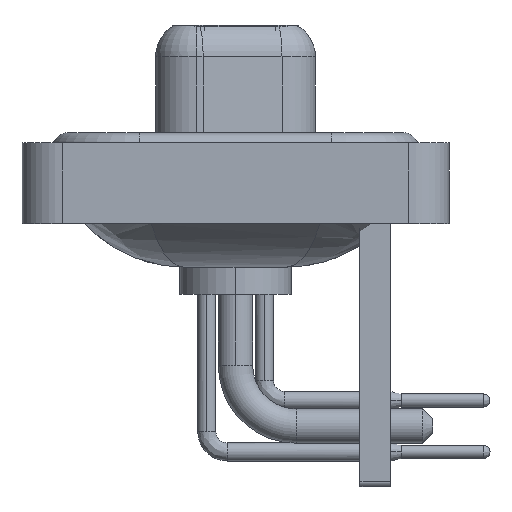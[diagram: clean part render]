
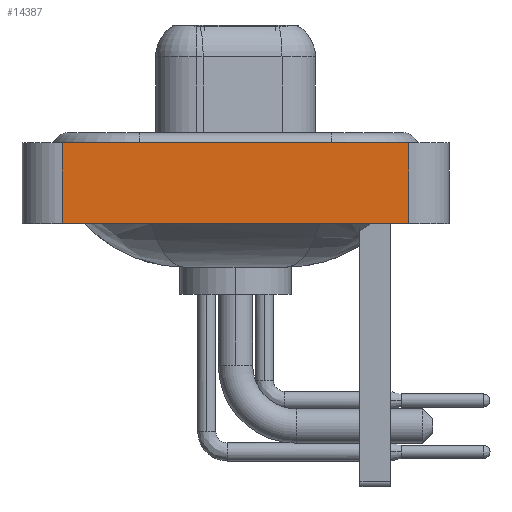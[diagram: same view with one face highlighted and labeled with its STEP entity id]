
A CAD part, left-side view. The second image highlights one B-rep face of the part: STEP entity #14387.
In plain terms, the highlighted planar face has unit normal (-1, 0, 0).
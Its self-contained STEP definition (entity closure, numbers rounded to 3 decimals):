
#184 = VECTOR ( 'NONE', #12606, 1000. ) ;
#1243 = DIRECTION ( 'NONE',  ( 0., -1., 0. ) ) ;
#2287 = LINE ( 'NONE', #10698, #6991 ) ;
#3509 = CARTESIAN_POINT ( 'NONE',  ( -7.35, -8.55, -3.6 ) ) ;
#3542 = CARTESIAN_POINT ( 'NONE',  ( -7.35, -8.55, -3.6 ) ) ;
#4070 = LINE ( 'NONE', #12712, #184 ) ;
#5156 = ORIENTED_EDGE ( 'NONE', *, *, #7178, .T. ) ;
#5842 = FACE_OUTER_BOUND ( 'NONE', #19448, .T. ) ;
#5980 = DIRECTION ( 'NONE',  ( 0., -1., 0. ) ) ;
#6646 = ORIENTED_EDGE ( 'NONE', *, *, #19752, .F. ) ;
#6935 = VERTEX_POINT ( 'NONE', #17417 ) ;
#6991 = VECTOR ( 'NONE', #5980, 1000. ) ;
#7178 = EDGE_CURVE ( 'NONE', #18136, #8039, #19956, .T. ) ;
#7414 = DIRECTION ( 'NONE',  ( 0., 0., 1. ) ) ;
#8039 = VERTEX_POINT ( 'NONE', #3509 ) ;
#9784 = CARTESIAN_POINT ( 'NONE',  ( -7.35, -8.55, -3.6 ) ) ;
#10698 = CARTESIAN_POINT ( 'NONE',  ( -7.35, -8.55, 0.4 ) ) ;
#11681 = CARTESIAN_POINT ( 'NONE',  ( -7.35, 8.55, 0.4 ) ) ;
#12059 = ORIENTED_EDGE ( 'NONE', *, *, #18385, .F. ) ;
#12606 = DIRECTION ( 'NONE',  ( 0., 0., 1. ) ) ;
#12712 = CARTESIAN_POINT ( 'NONE',  ( -7.35, 8.55, -3.6 ) ) ;
#12771 = ORIENTED_EDGE ( 'NONE', *, *, #13700, .T. ) ;
#13700 = EDGE_CURVE ( 'NONE', #8039, #6935, #20463, .T. ) ;
#14236 = PLANE ( 'NONE',  #20080 ) ;
#14387 = ADVANCED_FACE ( 'NONE', ( #5842 ), #14236, .T. ) ;
#14518 = VERTEX_POINT ( 'NONE', #11681 ) ;
#16012 = DIRECTION ( 'NONE',  ( -1., 0., 0. ) ) ;
#16272 = CARTESIAN_POINT ( 'NONE',  ( -7.35, 8.55, -3.6 ) ) ;
#17417 = CARTESIAN_POINT ( 'NONE',  ( -7.35, -8.55, 0.4 ) ) ;
#18136 = VERTEX_POINT ( 'NONE', #16272 ) ;
#18385 = EDGE_CURVE ( 'NONE', #18136, #14518, #4070, .T. ) ;
#18718 = VECTOR ( 'NONE', #18785, 1000. ) ;
#18785 = DIRECTION ( 'NONE',  ( 0., 0., 1. ) ) ;
#19206 = CARTESIAN_POINT ( 'NONE',  ( -7.35, -8.55, -3.6 ) ) ;
#19448 = EDGE_LOOP ( 'NONE', ( #12771, #6646, #12059, #5156 ) ) ;
#19752 = EDGE_CURVE ( 'NONE', #14518, #6935, #2287, .T. ) ;
#19956 = LINE ( 'NONE', #9784, #21800 ) ;
#20080 = AXIS2_PLACEMENT_3D ( 'NONE', #19206, #16012, #7414 ) ;
#20463 = LINE ( 'NONE', #3542, #18718 ) ;
#21800 = VECTOR ( 'NONE', #1243, 1000. ) ;
